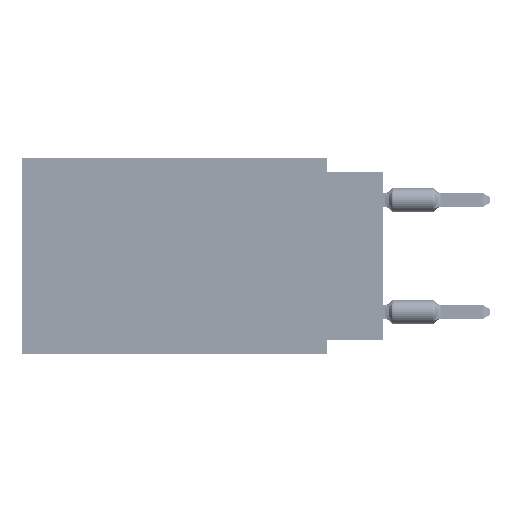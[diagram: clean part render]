
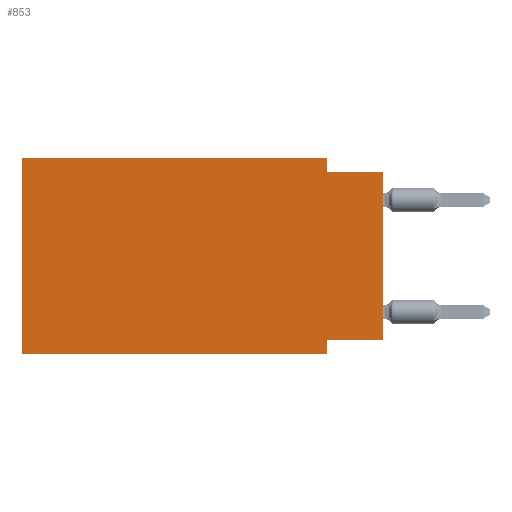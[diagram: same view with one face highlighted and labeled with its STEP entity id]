
A CAD part, left-side view. The second image highlights one B-rep face of the part: STEP entity #853.
In plain terms, the highlighted planar face has unit normal (-1, 0, 0).
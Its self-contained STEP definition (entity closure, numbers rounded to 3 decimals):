
#853 = ADVANCED_FACE ( 'NONE', ( #14141 ), #7360, .F. ) ;
#2184 = EDGE_CURVE ( 'NONE', #20753, #25944, #36730, .T. ) ;
#2506 = CARTESIAN_POINT ( 'NONE',  ( 0., 0., 0. ) ) ;
#2985 = VERTEX_POINT ( 'NONE', #30180 ) ;
#3081 = VECTOR ( 'NONE', #63365, 1000. ) ;
#4151 = DIRECTION ( 'NONE',  ( 0., -1., 0. ) ) ;
#5016 = DIRECTION ( 'NONE',  ( 0., 1., 0. ) ) ;
#7233 = EDGE_CURVE ( 'NONE', #34527, #13669, #57623, .T. ) ;
#7360 = PLANE ( 'NONE',  #8656 ) ;
#8656 = AXIS2_PLACEMENT_3D ( 'NONE', #83230, #42587, #70143 ) ;
#8864 = ORIENTED_EDGE ( 'NONE', *, *, #38983, .F. ) ;
#10539 = CARTESIAN_POINT ( 'NONE',  ( 0., 16.383, -8.89 ) ) ;
#12004 = VECTOR ( 'NONE', #71680, 1000. ) ;
#13669 = VERTEX_POINT ( 'NONE', #61573 ) ;
#14141 = FACE_OUTER_BOUND ( 'NONE', #46515, .T. ) ;
#14381 = VECTOR ( 'NONE', #4151, 1000. ) ;
#15050 = DIRECTION ( 'NONE',  ( 0., -1., 0. ) ) ;
#16667 = EDGE_CURVE ( 'NONE', #22281, #20753, #31457, .T. ) ;
#18885 = EDGE_CURVE ( 'NONE', #33769, #34527, #61013, .T. ) ;
#20753 = VERTEX_POINT ( 'NONE', #68410 ) ;
#21210 = ORIENTED_EDGE ( 'NONE', *, *, #47286, .T. ) ;
#22281 = VERTEX_POINT ( 'NONE', #10539 ) ;
#23815 = VECTOR ( 'NONE', #30961, 1000. ) ;
#24487 = ORIENTED_EDGE ( 'NONE', *, *, #2184, .F. ) ;
#25747 = ORIENTED_EDGE ( 'NONE', *, *, #43089, .T. ) ;
#25944 = VERTEX_POINT ( 'NONE', #75807 ) ;
#30180 = CARTESIAN_POINT ( 'NONE',  ( 0., 0., -0.635 ) ) ;
#30889 = VERTEX_POINT ( 'NONE', #62913 ) ;
#30961 = DIRECTION ( 'NONE',  ( 0., 0., -1. ) ) ;
#31457 = LINE ( 'NONE', #85664, #12004 ) ;
#31958 = VECTOR ( 'NONE', #63496, 1000. ) ;
#32547 = EDGE_CURVE ( 'NONE', #30889, #2985, #54376, .T. ) ;
#33615 = ORIENTED_EDGE ( 'NONE', *, *, #7233, .F. ) ;
#33769 = VERTEX_POINT ( 'NONE', #59125 ) ;
#34527 = VERTEX_POINT ( 'NONE', #45698 ) ;
#34930 = LINE ( 'NONE', #62471, #3081 ) ;
#36730 = LINE ( 'NONE', #72368, #14381 ) ;
#36839 = DIRECTION ( 'NONE',  ( 0., 0., 1. ) ) ;
#38203 = VECTOR ( 'NONE', #5016, 1000. ) ;
#38983 = EDGE_CURVE ( 'NONE', #25944, #30889, #34930, .T. ) ;
#42587 = DIRECTION ( 'NONE',  ( 1., 0., 0. ) ) ;
#43089 = EDGE_CURVE ( 'NONE', #22281, #13669, #43623, .T. ) ;
#43094 = ORIENTED_EDGE ( 'NONE', *, *, #16667, .F. ) ;
#43623 = LINE ( 'NONE', #77945, #31958 ) ;
#45698 = CARTESIAN_POINT ( 'NONE',  ( 0., 2.54, -8.255 ) ) ;
#46515 = EDGE_LOOP ( 'NONE', ( #21210, #87943, #8864, #24487, #43094, #25747, #33615, #48403 ) ) ;
#47286 = EDGE_CURVE ( 'NONE', #33769, #2985, #87660, .T. ) ;
#48403 = ORIENTED_EDGE ( 'NONE', *, *, #18885, .F. ) ;
#54376 = LINE ( 'NONE', #76470, #62970 ) ;
#57623 = LINE ( 'NONE', #84721, #23815 ) ;
#59125 = CARTESIAN_POINT ( 'NONE',  ( 0., 0., -8.255 ) ) ;
#61013 = LINE ( 'NONE', #67782, #38203 ) ;
#61573 = CARTESIAN_POINT ( 'NONE',  ( 0., 2.54, -8.89 ) ) ;
#62471 = CARTESIAN_POINT ( 'NONE',  ( 0., 2.54, 0. ) ) ;
#62913 = CARTESIAN_POINT ( 'NONE',  ( 0., 2.54, -0.635 ) ) ;
#62970 = VECTOR ( 'NONE', #15050, 1000. ) ;
#63365 = DIRECTION ( 'NONE',  ( 0., 0., -1. ) ) ;
#63496 = DIRECTION ( 'NONE',  ( 0., -1., 0. ) ) ;
#65840 = VECTOR ( 'NONE', #36839, 1000. ) ;
#67782 = CARTESIAN_POINT ( 'NONE',  ( 0., 0., -8.255 ) ) ;
#68410 = CARTESIAN_POINT ( 'NONE',  ( 0., 16.383, 0. ) ) ;
#70143 = DIRECTION ( 'NONE',  ( 0., 0., -1. ) ) ;
#71680 = DIRECTION ( 'NONE',  ( 0., 0., 1. ) ) ;
#72368 = CARTESIAN_POINT ( 'NONE',  ( 0., 16.383, 0. ) ) ;
#75807 = CARTESIAN_POINT ( 'NONE',  ( 0., 2.54, 0. ) ) ;
#76470 = CARTESIAN_POINT ( 'NONE',  ( 0., 0., -0.635 ) ) ;
#77945 = CARTESIAN_POINT ( 'NONE',  ( 0., 16.383, -8.89 ) ) ;
#83230 = CARTESIAN_POINT ( 'NONE',  ( 0., 16.383, 0. ) ) ;
#84721 = CARTESIAN_POINT ( 'NONE',  ( 0., 2.54, -8.89 ) ) ;
#85664 = CARTESIAN_POINT ( 'NONE',  ( 0., 16.383, 0. ) ) ;
#87660 = LINE ( 'NONE', #2506, #65840 ) ;
#87943 = ORIENTED_EDGE ( 'NONE', *, *, #32547, .F. ) ;
